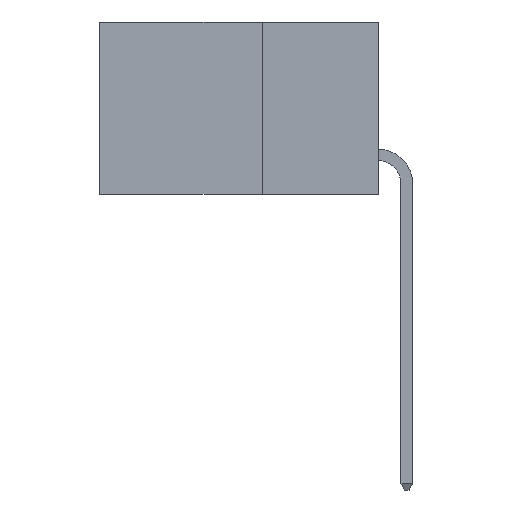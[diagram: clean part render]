
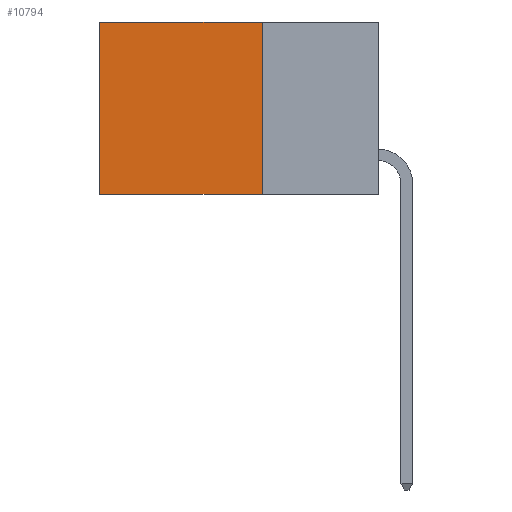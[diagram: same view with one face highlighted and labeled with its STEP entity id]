
A CAD part, left-side view. The second image highlights one B-rep face of the part: STEP entity #10794.
In plain terms, the highlighted planar face has unit normal (-1, 0, 0).
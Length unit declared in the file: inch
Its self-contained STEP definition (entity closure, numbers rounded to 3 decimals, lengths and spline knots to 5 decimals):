
#86 = AXIS2_PLACEMENT_3D ( 'NONE', #2954, #12057, #5346 ) ;
#218 = ORIENTED_EDGE ( 'NONE', *, *, #5129, .F. ) ;
#262 = ORIENTED_EDGE ( 'NONE', *, *, #6478, .F. ) ;
#507 = ORIENTED_EDGE ( 'NONE', *, *, #14477, .T. ) ;
#929 = EDGE_LOOP ( 'NONE', ( #9801, #218, #262, #507 ) ) ;
#2069 = FACE_OUTER_BOUND ( 'NONE', #929, .T. ) ;
#2110 = LINE ( 'NONE', #10840, #7607 ) ;
#2954 = CARTESIAN_POINT ( 'NONE',  ( 0.2615, 0.25, -0.37 ) ) ;
#3107 = CARTESIAN_POINT ( 'NONE',  ( 0.2615, 0.6, 0. ) ) ;
#3339 = CARTESIAN_POINT ( 'NONE',  ( 0.2615, 0.25, 0. ) ) ;
#3896 = VERTEX_POINT ( 'NONE', #8992 ) ;
#5129 = EDGE_CURVE ( 'NONE', #11907, #12974, #2110, .T. ) ;
#5346 = DIRECTION ( 'NONE',  ( 0., 0., -1. ) ) ;
#5543 = VECTOR ( 'NONE', #13870, 39.37008 ) ;
#5648 = VECTOR ( 'NONE', #14078, 39.37008 ) ;
#5740 = DIRECTION ( 'NONE',  ( 0., 1., 0. ) ) ;
#6478 = EDGE_CURVE ( 'NONE', #3896, #11907, #11860, .T. ) ;
#6594 = CARTESIAN_POINT ( 'NONE',  ( 0.2615, 0.6, -0.37 ) ) ;
#7197 = DIRECTION ( 'NONE',  ( 0., 1., 0. ) ) ;
#7607 = VECTOR ( 'NONE', #7197, 39.37008 ) ;
#8886 = EDGE_CURVE ( 'NONE', #10887, #12974, #14399, .T. ) ;
#8992 = CARTESIAN_POINT ( 'NONE',  ( 0.2615, 0.25, 0. ) ) ;
#9228 = VECTOR ( 'NONE', #5740, 39.37008 ) ;
#9801 = ORIENTED_EDGE ( 'NONE', *, *, #8886, .T. ) ;
#10633 = CARTESIAN_POINT ( 'NONE',  ( 0.2615, 0.25, -0.37 ) ) ;
#10794 = ADVANCED_FACE ( 'NONE', ( #2069 ), #10983, .F. ) ;
#10840 = CARTESIAN_POINT ( 'NONE',  ( 0.2615, 0.25, -0.37 ) ) ;
#10887 = VERTEX_POINT ( 'NONE', #3107 ) ;
#10983 = PLANE ( 'NONE',  #86 ) ;
#11860 = LINE ( 'NONE', #10633, #5543 ) ;
#11907 = VERTEX_POINT ( 'NONE', #13514 ) ;
#12057 = DIRECTION ( 'NONE',  ( 1., 0., 0. ) ) ;
#12754 = LINE ( 'NONE', #3339, #9228 ) ;
#12974 = VERTEX_POINT ( 'NONE', #6594 ) ;
#13019 = CARTESIAN_POINT ( 'NONE',  ( 0.2615, 0.6, -0.37 ) ) ;
#13514 = CARTESIAN_POINT ( 'NONE',  ( 0.2615, 0.25, -0.37 ) ) ;
#13870 = DIRECTION ( 'NONE',  ( 0., 0., -1. ) ) ;
#14078 = DIRECTION ( 'NONE',  ( 0., 0., -1. ) ) ;
#14399 = LINE ( 'NONE', #13019, #5648 ) ;
#14477 = EDGE_CURVE ( 'NONE', #3896, #10887, #12754, .T. ) ;
